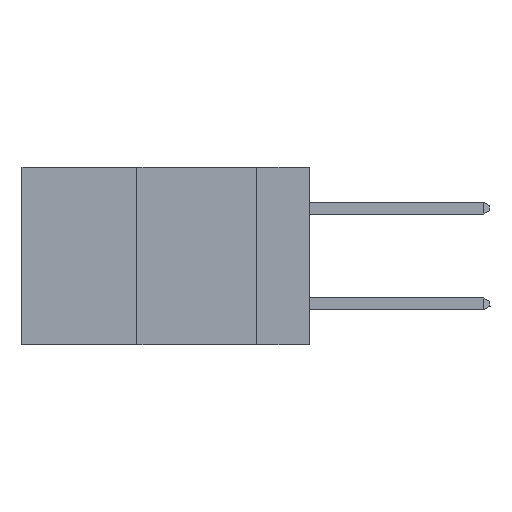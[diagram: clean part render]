
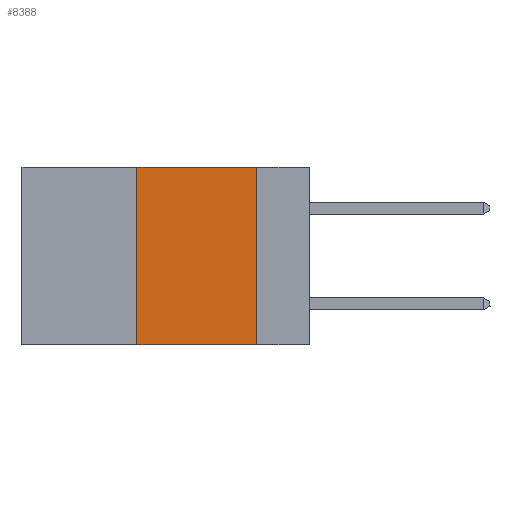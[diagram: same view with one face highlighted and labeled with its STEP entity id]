
A CAD part, left-side view. The second image highlights one B-rep face of the part: STEP entity #8388.
In plain terms, the highlighted planar face has unit normal (-1, 0, 0).
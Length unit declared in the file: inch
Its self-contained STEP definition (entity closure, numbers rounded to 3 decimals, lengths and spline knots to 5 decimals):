
#1055 = PLANE ( 'NONE',  #13194 ) ;
#2333 = DIRECTION ( 'NONE',  ( 0., -1., 0. ) ) ;
#3903 = FACE_OUTER_BOUND ( 'NONE', #23386, .T. ) ;
#4769 = CARTESIAN_POINT ( 'NONE',  ( 0., 0.6, 0. ) ) ;
#5672 = VECTOR ( 'NONE', #29155, 39.37008 ) ;
#6365 = CARTESIAN_POINT ( 'NONE',  ( 0., 0.36, 0. ) ) ;
#6957 = VERTEX_POINT ( 'NONE', #23977 ) ;
#7148 = LINE ( 'NONE', #30313, #24845 ) ;
#8388 = ADVANCED_FACE ( 'NONE', ( #3903 ), #1055, .F. ) ;
#8483 = ORIENTED_EDGE ( 'NONE', *, *, #17359, .F. ) ;
#11572 = VERTEX_POINT ( 'NONE', #32925 ) ;
#12517 = EDGE_CURVE ( 'NONE', #19358, #11572, #7148, .T. ) ;
#13194 = AXIS2_PLACEMENT_3D ( 'NONE', #4769, #32561, #19202 ) ;
#13725 = LINE ( 'NONE', #28342, #22820 ) ;
#14342 = CARTESIAN_POINT ( 'NONE',  ( 0., 0.36, 0. ) ) ;
#15098 = DIRECTION ( 'NONE',  ( 0., -1., 0. ) ) ;
#16410 = EDGE_CURVE ( 'NONE', #6957, #11572, #35189, .T. ) ;
#17359 = EDGE_CURVE ( 'NONE', #6957, #17495, #34639, .T. ) ;
#17495 = VERTEX_POINT ( 'NONE', #6365 ) ;
#19202 = DIRECTION ( 'NONE',  ( 0., 0., -1. ) ) ;
#19358 = VERTEX_POINT ( 'NONE', #31508 ) ;
#20796 = CARTESIAN_POINT ( 'NONE',  ( 0., 0.6, -0.37 ) ) ;
#21994 = VECTOR ( 'NONE', #15098, 39.37008 ) ;
#22441 = ORIENTED_EDGE ( 'NONE', *, *, #16410, .T. ) ;
#22820 = VECTOR ( 'NONE', #2333, 39.37008 ) ;
#23386 = EDGE_LOOP ( 'NONE', ( #29035, #35014, #8483, #22441 ) ) ;
#23977 = CARTESIAN_POINT ( 'NONE',  ( 0., 0.36, -0.37 ) ) ;
#24067 = DIRECTION ( 'NONE',  ( 0., 0., -1. ) ) ;
#24845 = VECTOR ( 'NONE', #24067, 39.37008 ) ;
#28342 = CARTESIAN_POINT ( 'NONE',  ( 0., 0.6, 0. ) ) ;
#29035 = ORIENTED_EDGE ( 'NONE', *, *, #12517, .F. ) ;
#29155 = DIRECTION ( 'NONE',  ( 0., 0., 1. ) ) ;
#29540 = EDGE_CURVE ( 'NONE', #17495, #19358, #13725, .T. ) ;
#30313 = CARTESIAN_POINT ( 'NONE',  ( 0., 0.11, 0. ) ) ;
#31508 = CARTESIAN_POINT ( 'NONE',  ( 0., 0.11, 0. ) ) ;
#32561 = DIRECTION ( 'NONE',  ( 1., 0., 0. ) ) ;
#32925 = CARTESIAN_POINT ( 'NONE',  ( 0., 0.11, -0.37 ) ) ;
#34639 = LINE ( 'NONE', #14342, #5672 ) ;
#35014 = ORIENTED_EDGE ( 'NONE', *, *, #29540, .F. ) ;
#35189 = LINE ( 'NONE', #20796, #21994 ) ;
